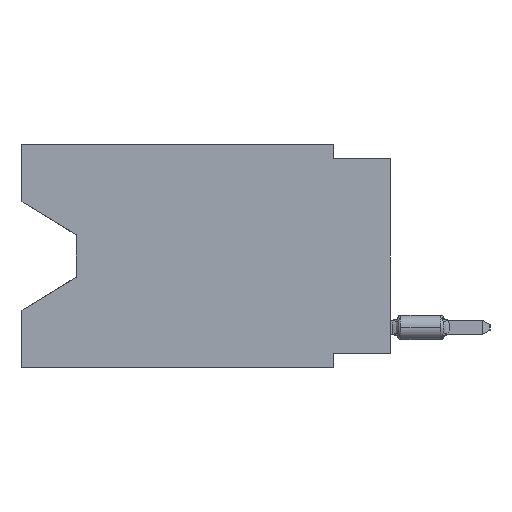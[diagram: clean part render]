
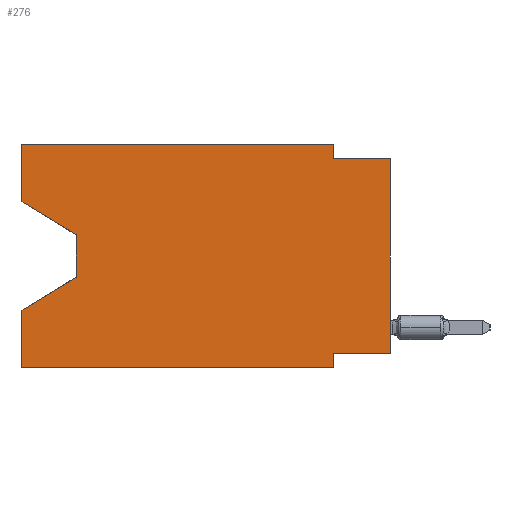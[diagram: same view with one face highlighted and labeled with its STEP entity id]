
A CAD part, left-side view. The second image highlights one B-rep face of the part: STEP entity #276.
In plain terms, the highlighted planar face has unit normal (-1, 0, 0).
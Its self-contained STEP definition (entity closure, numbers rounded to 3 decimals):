
#276 = ADVANCED_FACE ( 'NONE', ( #29135 ), #807, .F. ) ;
#481 = CARTESIAN_POINT ( 'NONE',  ( 0., 2.54, -9.906 ) ) ;
#507 = CARTESIAN_POINT ( 'NONE',  ( 0., 16.383, 0. ) ) ;
#573 = CARTESIAN_POINT ( 'NONE',  ( 0., 16.383, 0. ) ) ;
#807 = PLANE ( 'NONE',  #5540 ) ;
#1647 = VERTEX_POINT ( 'NONE', #20475 ) ;
#1792 = ORIENTED_EDGE ( 'NONE', *, *, #16184, .T. ) ;
#1864 = VERTEX_POINT ( 'NONE', #17654 ) ;
#1901 = VECTOR ( 'NONE', #21594, 1000. ) ;
#2315 = VERTEX_POINT ( 'NONE', #5710 ) ;
#2671 = VECTOR ( 'NONE', #20851, 1000. ) ;
#3292 = DIRECTION ( 'NONE',  ( 0., -1., 0. ) ) ;
#4584 = LINE ( 'NONE', #11843, #26897 ) ;
#4732 = DIRECTION ( 'NONE',  ( 0., 0.855, -0.519 ) ) ;
#5056 = VECTOR ( 'NONE', #11900, 1000. ) ;
#5252 = ORIENTED_EDGE ( 'NONE', *, *, #13608, .T. ) ;
#5540 = AXIS2_PLACEMENT_3D ( 'NONE', #15369, #17541, #17227 ) ;
#5657 = EDGE_CURVE ( 'NONE', #14010, #17399, #8939, .T. ) ;
#5710 = CARTESIAN_POINT ( 'NONE',  ( 0., 0., -9.271 ) ) ;
#6096 = VECTOR ( 'NONE', #6377, 1000. ) ;
#6377 = DIRECTION ( 'NONE',  ( 0., 0., 1. ) ) ;
#6392 = EDGE_CURVE ( 'NONE', #25202, #13642, #20625, .T. ) ;
#7119 = CARTESIAN_POINT ( 'NONE',  ( 0., 2.54, -9.906 ) ) ;
#7360 = CARTESIAN_POINT ( 'NONE',  ( 0., 16.383, -2.546 ) ) ;
#7369 = ORIENTED_EDGE ( 'NONE', *, *, #5657, .F. ) ;
#7401 = CARTESIAN_POINT ( 'NONE',  ( 0., 16.383, -9.906 ) ) ;
#7922 = LINE ( 'NONE', #481, #18604 ) ;
#8891 = ORIENTED_EDGE ( 'NONE', *, *, #24792, .F. ) ;
#8939 = LINE ( 'NONE', #10962, #2671 ) ;
#9158 = EDGE_CURVE ( 'NONE', #17146, #17393, #7922, .T. ) ;
#10094 = VERTEX_POINT ( 'NONE', #27761 ) ;
#10962 = CARTESIAN_POINT ( 'NONE',  ( 0., 2.54, 0. ) ) ;
#11175 = LINE ( 'NONE', #20468, #6096 ) ;
#11843 = CARTESIAN_POINT ( 'NONE',  ( 0., 13.97, -5.893 ) ) ;
#11900 = DIRECTION ( 'NONE',  ( 0., -1., 0. ) ) ;
#12551 = VECTOR ( 'NONE', #21142, 1000. ) ;
#12618 = VECTOR ( 'NONE', #22502, 1000. ) ;
#13096 = EDGE_LOOP ( 'NONE', ( #19945, #23523, #22360, #8891, #1792, #21510, #26273, #5252, #14063, #7369, #23764, #27576 ) ) ;
#13163 = CARTESIAN_POINT ( 'NONE',  ( 0., 2.54, -9.271 ) ) ;
#13608 = EDGE_CURVE ( 'NONE', #2315, #1864, #21188, .T. ) ;
#13642 = VERTEX_POINT ( 'NONE', #17623 ) ;
#14003 = VECTOR ( 'NONE', #14390, 1000. ) ;
#14010 = VERTEX_POINT ( 'NONE', #18680 ) ;
#14063 = ORIENTED_EDGE ( 'NONE', *, *, #19414, .F. ) ;
#14229 = CARTESIAN_POINT ( 'NONE',  ( 0., 0., 0. ) ) ;
#14390 = DIRECTION ( 'NONE',  ( 0., 0., 1. ) ) ;
#14842 = VECTOR ( 'NONE', #3292, 1000. ) ;
#15369 = CARTESIAN_POINT ( 'NONE',  ( 0., 16.383, 0. ) ) ;
#15487 = CARTESIAN_POINT ( 'NONE',  ( 0., 13.97, -4.013 ) ) ;
#15996 = CARTESIAN_POINT ( 'NONE',  ( 0., 0., -9.271 ) ) ;
#16184 = EDGE_CURVE ( 'NONE', #1647, #17393, #28149, .T. ) ;
#16666 = CARTESIAN_POINT ( 'NONE',  ( 0., 16.383, -2.546 ) ) ;
#17014 = CARTESIAN_POINT ( 'NONE',  ( 0., 2.54, -0.635 ) ) ;
#17111 = LINE ( 'NONE', #7360, #1901 ) ;
#17146 = VERTEX_POINT ( 'NONE', #13163 ) ;
#17227 = DIRECTION ( 'NONE',  ( 0., 0., -1. ) ) ;
#17363 = DIRECTION ( 'NONE',  ( 0., 0., -1. ) ) ;
#17393 = VERTEX_POINT ( 'NONE', #7119 ) ;
#17399 = VERTEX_POINT ( 'NONE', #17014 ) ;
#17541 = DIRECTION ( 'NONE',  ( 1., 0., 0. ) ) ;
#17623 = CARTESIAN_POINT ( 'NONE',  ( 0., 13.97, -5.893 ) ) ;
#17654 = CARTESIAN_POINT ( 'NONE',  ( 0., 0., -0.635 ) ) ;
#17742 = EDGE_CURVE ( 'NONE', #21843, #19338, #19125, .T. ) ;
#18270 = VECTOR ( 'NONE', #30220, 1000. ) ;
#18604 = VECTOR ( 'NONE', #17363, 1000. ) ;
#18680 = CARTESIAN_POINT ( 'NONE',  ( 0., 2.54, 0. ) ) ;
#19125 = LINE ( 'NONE', #24073, #12551 ) ;
#19338 = VERTEX_POINT ( 'NONE', #507 ) ;
#19414 = EDGE_CURVE ( 'NONE', #17399, #1864, #28992, .T. ) ;
#19945 = ORIENTED_EDGE ( 'NONE', *, *, #30619, .T. ) ;
#20194 = VECTOR ( 'NONE', #28908, 1000. ) ;
#20468 = CARTESIAN_POINT ( 'NONE',  ( 0., 16.383, 0. ) ) ;
#20475 = CARTESIAN_POINT ( 'NONE',  ( 0., 16.383, -9.906 ) ) ;
#20625 = LINE ( 'NONE', #24977, #12618 ) ;
#20798 = EDGE_CURVE ( 'NONE', #2315, #17146, #27748, .T. ) ;
#20851 = DIRECTION ( 'NONE',  ( 0., 0., -1. ) ) ;
#21142 = DIRECTION ( 'NONE',  ( 0., 0., 1. ) ) ;
#21188 = LINE ( 'NONE', #14229, #14003 ) ;
#21510 = ORIENTED_EDGE ( 'NONE', *, *, #9158, .F. ) ;
#21594 = DIRECTION ( 'NONE',  ( 0., -0.855, -0.519 ) ) ;
#21843 = VERTEX_POINT ( 'NONE', #16666 ) ;
#22360 = ORIENTED_EDGE ( 'NONE', *, *, #27636, .T. ) ;
#22502 = DIRECTION ( 'NONE',  ( 0., 0., -1. ) ) ;
#23523 = ORIENTED_EDGE ( 'NONE', *, *, #6392, .T. ) ;
#23764 = ORIENTED_EDGE ( 'NONE', *, *, #30245, .F. ) ;
#23804 = LINE ( 'NONE', #573, #20194 ) ;
#24073 = CARTESIAN_POINT ( 'NONE',  ( 0., 16.383, 0. ) ) ;
#24498 = CARTESIAN_POINT ( 'NONE',  ( 0., 0., -0.635 ) ) ;
#24792 = EDGE_CURVE ( 'NONE', #1647, #10094, #11175, .T. ) ;
#24977 = CARTESIAN_POINT ( 'NONE',  ( 0., 13.97, -4.013 ) ) ;
#25202 = VERTEX_POINT ( 'NONE', #15487 ) ;
#26273 = ORIENTED_EDGE ( 'NONE', *, *, #20798, .F. ) ;
#26897 = VECTOR ( 'NONE', #4732, 1000. ) ;
#27576 = ORIENTED_EDGE ( 'NONE', *, *, #17742, .F. ) ;
#27636 = EDGE_CURVE ( 'NONE', #13642, #10094, #4584, .T. ) ;
#27748 = LINE ( 'NONE', #15996, #18270 ) ;
#27761 = CARTESIAN_POINT ( 'NONE',  ( 0., 16.383, -7.36 ) ) ;
#28149 = LINE ( 'NONE', #7401, #5056 ) ;
#28908 = DIRECTION ( 'NONE',  ( 0., -1., 0. ) ) ;
#28992 = LINE ( 'NONE', #24498, #14842 ) ;
#29135 = FACE_OUTER_BOUND ( 'NONE', #13096, .T. ) ;
#30220 = DIRECTION ( 'NONE',  ( 0., 1., 0. ) ) ;
#30245 = EDGE_CURVE ( 'NONE', #19338, #14010, #23804, .T. ) ;
#30619 = EDGE_CURVE ( 'NONE', #21843, #25202, #17111, .T. ) ;
